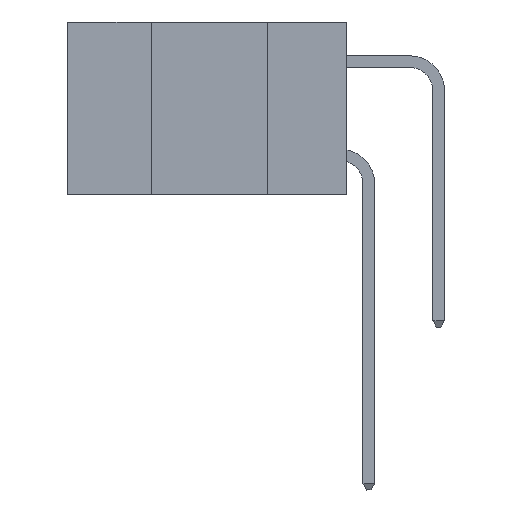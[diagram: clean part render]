
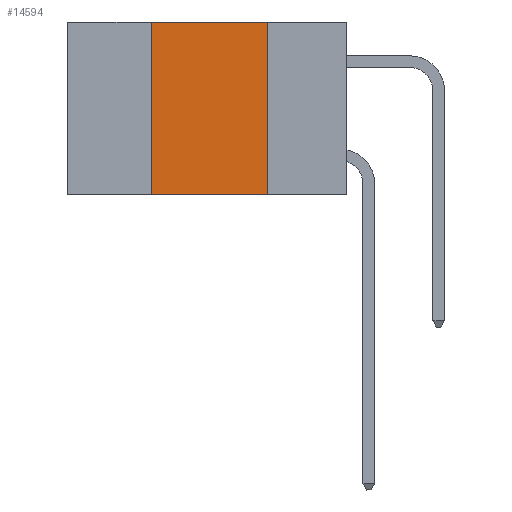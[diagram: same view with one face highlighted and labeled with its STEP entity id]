
A CAD part, left-side view. The second image highlights one B-rep face of the part: STEP entity #14594.
In plain terms, the highlighted planar face has unit normal (-1, 0, 0).
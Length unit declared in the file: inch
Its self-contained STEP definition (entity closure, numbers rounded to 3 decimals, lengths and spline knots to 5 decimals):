
#48 = LINE ( 'NONE', #21156, #5164 ) ;
#483 = EDGE_CURVE ( 'NONE', #1617, #2670, #25411, .T. ) ;
#1617 = VERTEX_POINT ( 'NONE', #9347 ) ;
#1845 = CARTESIAN_POINT ( 'NONE',  ( 0., 0.17, -0.37 ) ) ;
#1893 = DIRECTION ( 'NONE',  ( 1., 0., 0. ) ) ;
#2670 = VERTEX_POINT ( 'NONE', #15082 ) ;
#3588 = ORIENTED_EDGE ( 'NONE', *, *, #24922, .T. ) ;
#3700 = PLANE ( 'NONE',  #7819 ) ;
#3800 = VECTOR ( 'NONE', #27202, 39.37008 ) ;
#5164 = VECTOR ( 'NONE', #16764, 39.37008 ) ;
#6163 = LINE ( 'NONE', #9752, #3800 ) ;
#7819 = AXIS2_PLACEMENT_3D ( 'NONE', #19029, #1893, #15106 ) ;
#9347 = CARTESIAN_POINT ( 'NONE',  ( 0., 0.42, -0.37 ) ) ;
#9596 = LINE ( 'NONE', #15344, #20498 ) ;
#9610 = EDGE_CURVE ( 'NONE', #23715, #19481, #48, .T. ) ;
#9752 = CARTESIAN_POINT ( 'NONE',  ( 0., 0.6, -0.37 ) ) ;
#9899 = CARTESIAN_POINT ( 'NONE',  ( 0., 0.17, 0. ) ) ;
#10002 = ORIENTED_EDGE ( 'NONE', *, *, #21633, .F. ) ;
#11411 = CARTESIAN_POINT ( 'NONE',  ( 0., 0.42, 0. ) ) ;
#13963 = FACE_OUTER_BOUND ( 'NONE', #16446, .T. ) ;
#14594 = ADVANCED_FACE ( 'NONE', ( #13963 ), #3700, .F. ) ;
#15082 = CARTESIAN_POINT ( 'NONE',  ( 0., 0.42, 0. ) ) ;
#15106 = DIRECTION ( 'NONE',  ( 0., 0., -1. ) ) ;
#15344 = CARTESIAN_POINT ( 'NONE',  ( 0., 0.6, 0. ) ) ;
#16247 = ORIENTED_EDGE ( 'NONE', *, *, #483, .F. ) ;
#16446 = EDGE_LOOP ( 'NONE', ( #23461, #10002, #16247, #3588 ) ) ;
#16764 = DIRECTION ( 'NONE',  ( 0., 0., -1. ) ) ;
#17825 = DIRECTION ( 'NONE',  ( 0., -1., 0. ) ) ;
#19029 = CARTESIAN_POINT ( 'NONE',  ( 0., 0.6, 0. ) ) ;
#19481 = VERTEX_POINT ( 'NONE', #1845 ) ;
#20154 = DIRECTION ( 'NONE',  ( 0., 0., 1. ) ) ;
#20498 = VECTOR ( 'NONE', #17825, 39.37008 ) ;
#21156 = CARTESIAN_POINT ( 'NONE',  ( 0., 0.17, 0. ) ) ;
#21633 = EDGE_CURVE ( 'NONE', #2670, #23715, #9596, .T. ) ;
#23023 = VECTOR ( 'NONE', #20154, 39.37008 ) ;
#23461 = ORIENTED_EDGE ( 'NONE', *, *, #9610, .F. ) ;
#23715 = VERTEX_POINT ( 'NONE', #9899 ) ;
#24922 = EDGE_CURVE ( 'NONE', #1617, #19481, #6163, .T. ) ;
#25411 = LINE ( 'NONE', #11411, #23023 ) ;
#27202 = DIRECTION ( 'NONE',  ( 0., -1., 0. ) ) ;
